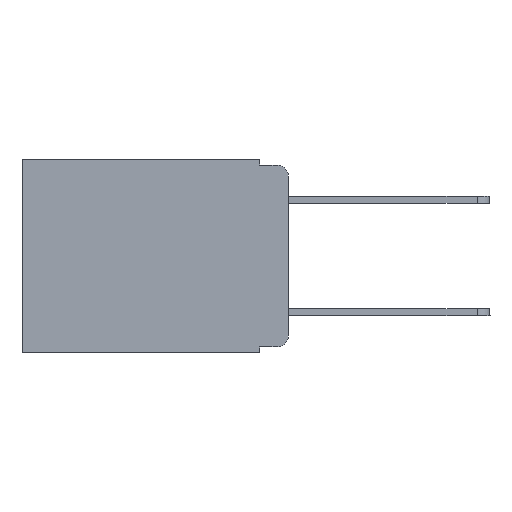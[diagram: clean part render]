
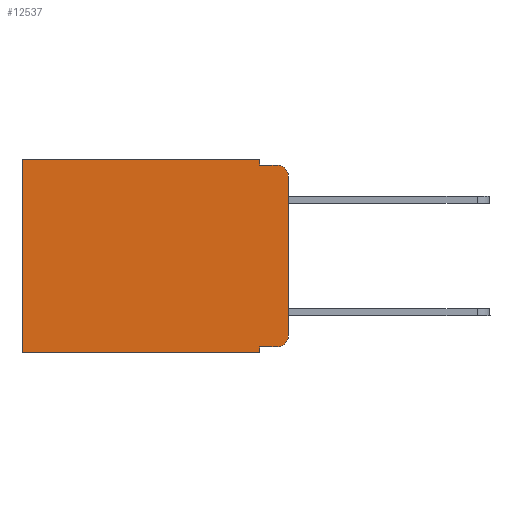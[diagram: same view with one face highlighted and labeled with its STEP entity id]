
A CAD part, left-side view. The second image highlights one B-rep face of the part: STEP entity #12537.
In plain terms, the highlighted planar face has unit normal (-1, 0, 0).
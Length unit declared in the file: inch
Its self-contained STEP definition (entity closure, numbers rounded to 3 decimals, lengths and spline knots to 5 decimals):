
#139 = VECTOR ( 'NONE', #23165, 39.37008 ) ;
#418 = VERTEX_POINT ( 'NONE', #13402 ) ;
#1300 = CARTESIAN_POINT ( 'NONE',  ( 0.298, 0., -0.313 ) ) ;
#1427 = ORIENTED_EDGE ( 'NONE', *, *, #7902, .T. ) ;
#1464 = CARTESIAN_POINT ( 'NONE',  ( 0.298, 0.051, -0.343 ) ) ;
#1471 = VERTEX_POINT ( 'NONE', #23486 ) ;
#1761 = VECTOR ( 'NONE', #15371, 39.37008 ) ;
#1902 = LINE ( 'NONE', #9688, #23866 ) ;
#2075 = VERTEX_POINT ( 'NONE', #2761 ) ;
#2487 = EDGE_CURVE ( 'NONE', #14575, #13186, #13401, .T. ) ;
#2694 = CARTESIAN_POINT ( 'NONE',  ( 0.298, 0., 0. ) ) ;
#2703 = CARTESIAN_POINT ( 'NONE',  ( 0.298, 0.02, -0.333 ) ) ;
#2761 = CARTESIAN_POINT ( 'NONE',  ( 0.298, 0., -0.03 ) ) ;
#2989 = DIRECTION ( 'NONE',  ( 0., -1., 0. ) ) ;
#3059 = DIRECTION ( 'NONE',  ( 0., 0., -1. ) ) ;
#3368 = AXIS2_PLACEMENT_3D ( 'NONE', #24048, #12499, #3059 ) ;
#3400 = ORIENTED_EDGE ( 'NONE', *, *, #2487, .T. ) ;
#3667 = VERTEX_POINT ( 'NONE', #12190 ) ;
#3747 = DIRECTION ( 'NONE',  ( 0., 1., 0. ) ) ;
#3765 = ORIENTED_EDGE ( 'NONE', *, *, #5130, .T. ) ;
#3783 = LINE ( 'NONE', #21253, #1761 ) ;
#4089 = ORIENTED_EDGE ( 'NONE', *, *, #15501, .T. ) ;
#4182 = EDGE_CURVE ( 'NONE', #1471, #22203, #12796, .T. ) ;
#4320 = LINE ( 'NONE', #9621, #139 ) ;
#5068 = EDGE_CURVE ( 'NONE', #418, #3667, #6811, .T. ) ;
#5130 = EDGE_CURVE ( 'NONE', #2075, #22203, #21334, .T. ) ;
#5247 = DIRECTION ( 'NONE',  ( 1., 0., 0. ) ) ;
#5376 = VERTEX_POINT ( 'NONE', #11579 ) ;
#5618 = DIRECTION ( 'NONE',  ( 0., 0., -1. ) ) ;
#5951 = VECTOR ( 'NONE', #3747, 39.37008 ) ;
#6811 = LINE ( 'NONE', #2694, #14121 ) ;
#7309 = DIRECTION ( 'NONE',  ( -1., 0., 0. ) ) ;
#7354 = CARTESIAN_POINT ( 'NONE',  ( 0.298, 0., 0. ) ) ;
#7500 = CARTESIAN_POINT ( 'NONE',  ( 0.298, 0., 0. ) ) ;
#7902 = EDGE_CURVE ( 'NONE', #3667, #18767, #4320, .T. ) ;
#9088 = CARTESIAN_POINT ( 'NONE',  ( 0.298, 0.473, -0.343 ) ) ;
#9267 = DIRECTION ( 'NONE',  ( 0., 0., -1. ) ) ;
#9398 = FACE_OUTER_BOUND ( 'NONE', #19717, .T. ) ;
#9404 = ORIENTED_EDGE ( 'NONE', *, *, #15152, .F. ) ;
#9621 = CARTESIAN_POINT ( 'NONE',  ( 0.298, 0.473, 0. ) ) ;
#9688 = CARTESIAN_POINT ( 'NONE',  ( 0.298, 0.051, 0. ) ) ;
#10508 = AXIS2_PLACEMENT_3D ( 'NONE', #18643, #7309, #12976 ) ;
#10953 = CARTESIAN_POINT ( 'NONE',  ( 0.298, 0.02, -0.01 ) ) ;
#11299 = EDGE_CURVE ( 'NONE', #418, #1471, #1902, .T. ) ;
#11579 = CARTESIAN_POINT ( 'NONE',  ( 0.298, 0.051, -0.333 ) ) ;
#11621 = LINE ( 'NONE', #24695, #18053 ) ;
#12190 = CARTESIAN_POINT ( 'NONE',  ( 0.298, 0.473, 0. ) ) ;
#12499 = DIRECTION ( 'NONE',  ( -1., 0., 0. ) ) ;
#12537 = ADVANCED_FACE ( 'NONE', ( #9398 ), #24710, .F. ) ;
#12796 = LINE ( 'NONE', #14828, #17856 ) ;
#12976 = DIRECTION ( 'NONE',  ( 0., 0., -1. ) ) ;
#13186 = VERTEX_POINT ( 'NONE', #1300 ) ;
#13276 = LINE ( 'NONE', #7354, #22768 ) ;
#13401 = CIRCLE ( 'NONE', #3368, 0.02 ) ;
#13402 = CARTESIAN_POINT ( 'NONE',  ( 0.298, 0.051, 0. ) ) ;
#13702 = DIRECTION ( 'NONE',  ( 0., 0., -1. ) ) ;
#14121 = VECTOR ( 'NONE', #24161, 39.37008 ) ;
#14575 = VERTEX_POINT ( 'NONE', #2703 ) ;
#14828 = CARTESIAN_POINT ( 'NONE',  ( 0.298, 0.051, -0.01 ) ) ;
#14857 = ORIENTED_EDGE ( 'NONE', *, *, #11299, .F. ) ;
#15049 = ORIENTED_EDGE ( 'NONE', *, *, #4182, .F. ) ;
#15152 = EDGE_CURVE ( 'NONE', #16922, #18767, #17341, .T. ) ;
#15371 = DIRECTION ( 'NONE',  ( 0., 0., -1. ) ) ;
#15501 = EDGE_CURVE ( 'NONE', #5376, #14575, #11621, .T. ) ;
#16922 = VERTEX_POINT ( 'NONE', #1464 ) ;
#17341 = LINE ( 'NONE', #19321, #5951 ) ;
#17856 = VECTOR ( 'NONE', #2989, 39.37008 ) ;
#17875 = ORIENTED_EDGE ( 'NONE', *, *, #5068, .T. ) ;
#18053 = VECTOR ( 'NONE', #21052, 39.37008 ) ;
#18643 = CARTESIAN_POINT ( 'NONE',  ( 0.298, 0.02, -0.03 ) ) ;
#18767 = VERTEX_POINT ( 'NONE', #9088 ) ;
#18913 = ORIENTED_EDGE ( 'NONE', *, *, #22691, .F. ) ;
#18926 = EDGE_CURVE ( 'NONE', #5376, #16922, #3783, .T. ) ;
#19321 = CARTESIAN_POINT ( 'NONE',  ( 0.298, 0., -0.343 ) ) ;
#19717 = EDGE_LOOP ( 'NONE', ( #18913, #3765, #15049, #14857, #17875, #1427, #9404, #24786, #4089, #3400 ) ) ;
#21052 = DIRECTION ( 'NONE',  ( 0., -1., 0. ) ) ;
#21253 = CARTESIAN_POINT ( 'NONE',  ( 0.298, 0.051, 0. ) ) ;
#21334 = CIRCLE ( 'NONE', #10508, 0.02 ) ;
#22203 = VERTEX_POINT ( 'NONE', #10953 ) ;
#22691 = EDGE_CURVE ( 'NONE', #2075, #13186, #13276, .T. ) ;
#22768 = VECTOR ( 'NONE', #9267, 39.37008 ) ;
#23165 = DIRECTION ( 'NONE',  ( 0., 0., -1. ) ) ;
#23486 = CARTESIAN_POINT ( 'NONE',  ( 0.298, 0.051, -0.01 ) ) ;
#23866 = VECTOR ( 'NONE', #13702, 39.37008 ) ;
#23931 = AXIS2_PLACEMENT_3D ( 'NONE', #7500, #5247, #5618 ) ;
#24048 = CARTESIAN_POINT ( 'NONE',  ( 0.298, 0.02, -0.313 ) ) ;
#24161 = DIRECTION ( 'NONE',  ( 0., 1., 0. ) ) ;
#24695 = CARTESIAN_POINT ( 'NONE',  ( 0.298, 0.051, -0.333 ) ) ;
#24710 = PLANE ( 'NONE',  #23931 ) ;
#24786 = ORIENTED_EDGE ( 'NONE', *, *, #18926, .F. ) ;
